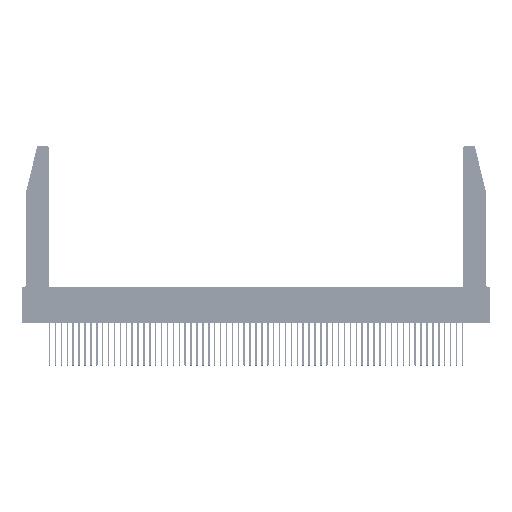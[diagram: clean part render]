
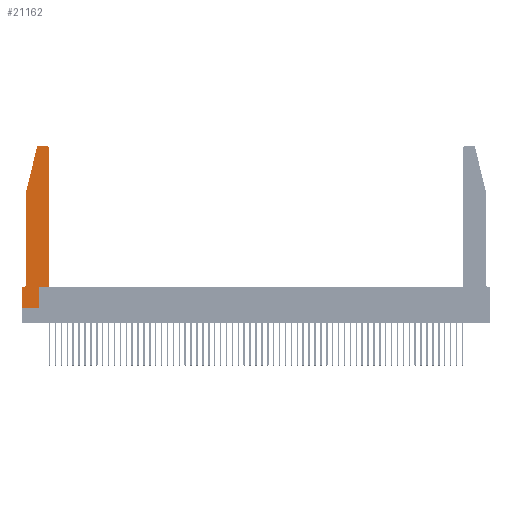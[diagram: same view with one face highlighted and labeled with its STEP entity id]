
A CAD part, top view. The second image highlights one B-rep face of the part: STEP entity #21162.
In plain terms, the highlighted planar face has unit normal (0, 0, 1).
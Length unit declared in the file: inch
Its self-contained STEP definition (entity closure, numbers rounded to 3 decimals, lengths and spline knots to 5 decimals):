
#631 = ORIENTED_EDGE ( 'NONE', *, *, #26633, .T. ) ;
#716 = CARTESIAN_POINT ( 'NONE',  ( 0.4505, 2.72, 0.37 ) ) ;
#786 = CARTESIAN_POINT ( 'NONE',  ( 0., 0.35, 0.37 ) ) ;
#1000 = VERTEX_POINT ( 'NONE', #716 ) ;
#1763 = ORIENTED_EDGE ( 'NONE', *, *, #17830, .T. ) ;
#2214 = ORIENTED_EDGE ( 'NONE', *, *, #26816, .T. ) ;
#2237 = VECTOR ( 'NONE', #12430, 39.37008 ) ;
#2259 = CARTESIAN_POINT ( 'NONE',  ( 0.0755, 2., 0.37 ) ) ;
#2506 = ORIENTED_EDGE ( 'NONE', *, *, #50781, .T. ) ;
#2795 = DIRECTION ( 'NONE',  ( 0., 0., -1. ) ) ;
#3738 = EDGE_CURVE ( 'NONE', #41133, #5930, #32220, .T. ) ;
#4061 = LINE ( 'NONE', #46230, #27276 ) ;
#4689 = DIRECTION ( 'NONE',  ( 1., 0., 0. ) ) ;
#4871 = CARTESIAN_POINT ( 'NONE',  ( 0.4505, 0.35, 0.37 ) ) ;
#4881 = CARTESIAN_POINT ( 'NONE',  ( 0.4205, 2.72, 0.37 ) ) ;
#5196 = DIRECTION ( 'NONE',  ( 0., -1., 0. ) ) ;
#5368 = CARTESIAN_POINT ( 'NONE',  ( 0.284, 2.75, 0.37 ) ) ;
#5862 = ORIENTED_EDGE ( 'NONE', *, *, #27819, .T. ) ;
#5930 = VERTEX_POINT ( 'NONE', #9674 ) ;
#7126 = CARTESIAN_POINT ( 'NONE',  ( 0.2865, 0.35, 0.37 ) ) ;
#7406 = DIRECTION ( 'NONE',  ( -1., 0., 0. ) ) ;
#7990 = CARTESIAN_POINT ( 'NONE',  ( 0.4505, 0.35, 0.37 ) ) ;
#8853 = CARTESIAN_POINT ( 'NONE',  ( 0.25487, 2.72718, 0.37 ) ) ;
#9602 = DIRECTION ( 'NONE',  ( -1., 0., 0. ) ) ;
#9674 = CARTESIAN_POINT ( 'NONE',  ( 0.2865, 0.35, 0.37 ) ) ;
#9722 = CARTESIAN_POINT ( 'NONE',  ( 0.4205, 2.75, 0.37 ) ) ;
#11221 = CARTESIAN_POINT ( 'NONE',  ( 0.2605, 2.75, 0.37 ) ) ;
#11586 = VERTEX_POINT ( 'NONE', #786 ) ;
#12430 = DIRECTION ( 'NONE',  ( 1., 0., 0. ) ) ;
#12446 = LINE ( 'NONE', #38077, #30202 ) ;
#13183 = VERTEX_POINT ( 'NONE', #8853 ) ;
#13627 = CARTESIAN_POINT ( 'NONE',  ( 0.2865, 0., 0.37 ) ) ;
#13868 = LINE ( 'NONE', #47392, #2237 ) ;
#15742 = AXIS2_PLACEMENT_3D ( 'NONE', #4881, #34707, #4689 ) ;
#15971 = CARTESIAN_POINT ( 'NONE',  ( 0.0755, 0.42, 0.37 ) ) ;
#15997 = DIRECTION ( 'NONE',  ( 1., 0., 0. ) ) ;
#16620 = VERTEX_POINT ( 'NONE', #32236 ) ;
#17382 = VECTOR ( 'NONE', #5196, 39.37008 ) ;
#17829 = EDGE_CURVE ( 'NONE', #22925, #13183, #28307, .T. ) ;
#17830 = EDGE_CURVE ( 'NONE', #11586, #16620, #42042, .T. ) ;
#18722 = CARTESIAN_POINT ( 'NONE',  ( 0.284, 2.72, 0.37 ) ) ;
#18992 = DIRECTION ( 'NONE',  ( 0., -1., 0. ) ) ;
#19245 = VECTOR ( 'NONE', #35062, 39.37008 ) ;
#19249 = VERTEX_POINT ( 'NONE', #2259 ) ;
#19603 = DIRECTION ( 'NONE',  ( -1., 0., 0. ) ) ;
#19736 = ORIENTED_EDGE ( 'NONE', *, *, #36548, .T. ) ;
#21162 = ADVANCED_FACE ( 'NONE', ( #55883 ), #51554, .T. ) ;
#22900 = CIRCLE ( 'NONE', #26421, 0.07 ) ;
#22925 = VERTEX_POINT ( 'NONE', #5368 ) ;
#23539 = EDGE_LOOP ( 'NONE', ( #30746, #32248, #28650, #2214, #2506, #43343, #1763, #19736, #44564, #5862, #54228, #631 ) ) ;
#23937 = CIRCLE ( 'NONE', #15742, 0.03 ) ;
#24860 = EDGE_CURVE ( 'NONE', #39183, #1000, #30892, .T. ) ;
#25019 = DIRECTION ( 'NONE',  ( -0.239, -0.971, 0. ) ) ;
#26421 = AXIS2_PLACEMENT_3D ( 'NONE', #33552, #2795, #7406 ) ;
#26633 = EDGE_CURVE ( 'NONE', #1000, #52878, #23937, .T. ) ;
#26816 = EDGE_CURVE ( 'NONE', #19249, #45634, #48621, .T. ) ;
#27276 = VECTOR ( 'NONE', #50644, 39.37008 ) ;
#27819 = EDGE_CURVE ( 'NONE', #5930, #39183, #4061, .T. ) ;
#28307 = CIRCLE ( 'NONE', #51315, 0.03 ) ;
#28451 = VECTOR ( 'NONE', #19603, 39.37008 ) ;
#28650 = ORIENTED_EDGE ( 'NONE', *, *, #41511, .T. ) ;
#29059 = DIRECTION ( 'NONE',  ( 0., 1., 0. ) ) ;
#30190 = LINE ( 'NONE', #37869, #41836 ) ;
#30202 = VECTOR ( 'NONE', #9602, 39.37008 ) ;
#30347 = EDGE_CURVE ( 'NONE', #52878, #22925, #51714, .T. ) ;
#30746 = ORIENTED_EDGE ( 'NONE', *, *, #30347, .T. ) ;
#30892 = LINE ( 'NONE', #4871, #19245 ) ;
#32101 = DIRECTION ( 'NONE',  ( 1., 0., 0. ) ) ;
#32220 = LINE ( 'NONE', #7126, #40418 ) ;
#32236 = CARTESIAN_POINT ( 'NONE',  ( 0., 0., 0.37 ) ) ;
#32248 = ORIENTED_EDGE ( 'NONE', *, *, #17829, .T. ) ;
#33552 = CARTESIAN_POINT ( 'NONE',  ( 0.0055, 0.42, 0.37 ) ) ;
#34275 = AXIS2_PLACEMENT_3D ( 'NONE', #47156, #55200, #15997 ) ;
#34707 = DIRECTION ( 'NONE',  ( 0., 0., 1. ) ) ;
#35062 = DIRECTION ( 'NONE',  ( 0., 1., 0. ) ) ;
#36271 = VERTEX_POINT ( 'NONE', #49533 ) ;
#36548 = EDGE_CURVE ( 'NONE', #16620, #41133, #13868, .T. ) ;
#37869 = CARTESIAN_POINT ( 'NONE',  ( 0.0755, 2., 0.37 ) ) ;
#38077 = CARTESIAN_POINT ( 'NONE',  ( 0.0755, 0.35, 0.37 ) ) ;
#39183 = VERTEX_POINT ( 'NONE', #7990 ) ;
#40163 = DIRECTION ( 'NONE',  ( 0., 0., 1. ) ) ;
#40418 = VECTOR ( 'NONE', #29059, 39.37008 ) ;
#41133 = VERTEX_POINT ( 'NONE', #13627 ) ;
#41511 = EDGE_CURVE ( 'NONE', #13183, #19249, #30190, .T. ) ;
#41836 = VECTOR ( 'NONE', #25019, 39.37008 ) ;
#42042 = LINE ( 'NONE', #49116, #17382 ) ;
#43343 = ORIENTED_EDGE ( 'NONE', *, *, #53875, .T. ) ;
#44564 = ORIENTED_EDGE ( 'NONE', *, *, #3738, .T. ) ;
#45634 = VERTEX_POINT ( 'NONE', #15971 ) ;
#46230 = CARTESIAN_POINT ( 'NONE',  ( 0.4505, 0.35, 0.37 ) ) ;
#47156 = CARTESIAN_POINT ( 'NONE',  ( 0., 0.35, 0.37 ) ) ;
#47392 = CARTESIAN_POINT ( 'NONE',  ( 0., 0., 0.37 ) ) ;
#48621 = LINE ( 'NONE', #53772, #54110 ) ;
#49116 = CARTESIAN_POINT ( 'NONE',  ( 0., 0., 0.37 ) ) ;
#49533 = CARTESIAN_POINT ( 'NONE',  ( 0.0055, 0.35, 0.37 ) ) ;
#50644 = DIRECTION ( 'NONE',  ( 1., 0., 0. ) ) ;
#50781 = EDGE_CURVE ( 'NONE', #45634, #36271, #22900, .T. ) ;
#51315 = AXIS2_PLACEMENT_3D ( 'NONE', #18722, #40163, #32101 ) ;
#51554 = PLANE ( 'NONE',  #34275 ) ;
#51714 = LINE ( 'NONE', #11221, #28451 ) ;
#52878 = VERTEX_POINT ( 'NONE', #9722 ) ;
#53772 = CARTESIAN_POINT ( 'NONE',  ( 0.0755, 2., 0.37 ) ) ;
#53875 = EDGE_CURVE ( 'NONE', #36271, #11586, #12446, .T. ) ;
#54110 = VECTOR ( 'NONE', #18992, 39.37008 ) ;
#54228 = ORIENTED_EDGE ( 'NONE', *, *, #24860, .T. ) ;
#55200 = DIRECTION ( 'NONE',  ( 0., 0., 1. ) ) ;
#55883 = FACE_OUTER_BOUND ( 'NONE', #23539, .T. ) ;
